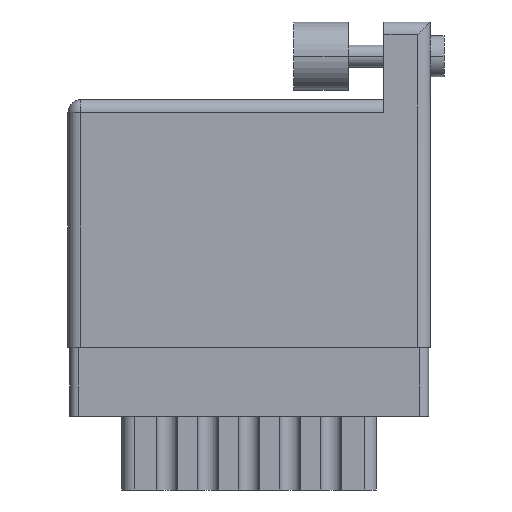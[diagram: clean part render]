
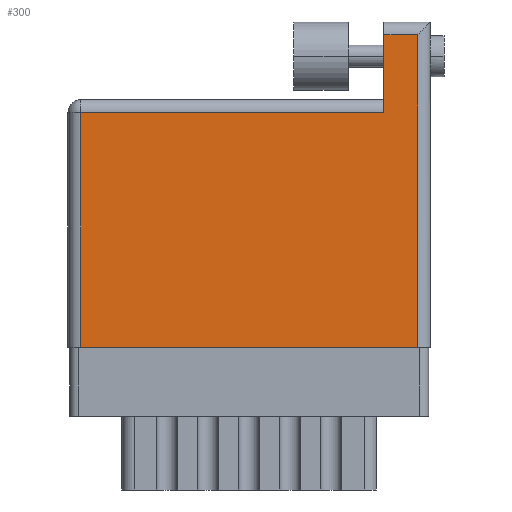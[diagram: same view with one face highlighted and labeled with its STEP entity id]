
A CAD part, front view. The second image highlights one B-rep face of the part: STEP entity #300.
In plain terms, the highlighted face is planar.
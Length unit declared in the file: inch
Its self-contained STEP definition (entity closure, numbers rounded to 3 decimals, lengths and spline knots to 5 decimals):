
#2 = EDGE_CURVE ( 'NONE', #20556, #6026, #22834, .T. ) ;
#300 = ADVANCED_FACE ( 'NONE', ( #23068 ), #21240, .F. ) ;
#415 = ORIENTED_EDGE ( 'NONE', *, *, #13060, .T. ) ;
#594 = ORIENTED_EDGE ( 'NONE', *, *, #13523, .T. ) ;
#717 = ORIENTED_EDGE ( 'NONE', *, *, #2, .T. ) ;
#747 = VERTEX_POINT ( 'NONE', #3722 ) ;
#860 = LINE ( 'NONE', #8814, #20825 ) ;
#861 = LINE ( 'NONE', #2825, #14377 ) ;
#1344 = CARTESIAN_POINT ( 'NONE',  ( 1.155, 1.143, 0. ) ) ;
#1996 = CARTESIAN_POINT ( 'NONE',  ( 1.278, 1.143, 0. ) ) ;
#2564 = DIRECTION ( 'NONE',  ( -1., 0., 0. ) ) ;
#2669 = VERTEX_POINT ( 'NONE', #22211 ) ;
#2825 = CARTESIAN_POINT ( 'NONE',  ( 0., 0.859, 0. ) ) ;
#2884 = LINE ( 'NONE', #23186, #16042 ) ;
#2885 = VERTEX_POINT ( 'NONE', #1996 ) ;
#3379 = VERTEX_POINT ( 'NONE', #1344 ) ;
#3722 = CARTESIAN_POINT ( 'NONE',  ( 0.047, 0.859, 0. ) ) ;
#4120 = VECTOR ( 'NONE', #13443, 39.37008 ) ;
#4648 = CARTESIAN_POINT ( 'NONE',  ( 0.047, 0., 0. ) ) ;
#4870 = DIRECTION ( 'NONE',  ( 1., 0., 0. ) ) ;
#5479 = CARTESIAN_POINT ( 'NONE',  ( 1.155, 1.143, 0. ) ) ;
#6026 = VERTEX_POINT ( 'NONE', #14923 ) ;
#7432 = DIRECTION ( 'NONE',  ( 0., 0., -1. ) ) ;
#8174 = EDGE_LOOP ( 'NONE', ( #717, #17718, #594, #415, #17998, #18497 ) ) ;
#8814 = CARTESIAN_POINT ( 'NONE',  ( 1.155, 1.19, 0. ) ) ;
#11611 = CARTESIAN_POINT ( 'NONE',  ( 0., 0.906, 0. ) ) ;
#13060 = EDGE_CURVE ( 'NONE', #3379, #2669, #860, .T. ) ;
#13111 = VECTOR ( 'NONE', #4870, 39.37008 ) ;
#13193 = DIRECTION ( 'NONE',  ( -1., 0., 0. ) ) ;
#13443 = DIRECTION ( 'NONE',  ( -1., 0., 0. ) ) ;
#13523 = EDGE_CURVE ( 'NONE', #2885, #3379, #23319, .T. ) ;
#14261 = EDGE_CURVE ( 'NONE', #747, #20556, #20016, .T. ) ;
#14377 = VECTOR ( 'NONE', #2564, 39.37008 ) ;
#14923 = CARTESIAN_POINT ( 'NONE',  ( 1.278, 0., 0. ) ) ;
#16042 = VECTOR ( 'NONE', #16691, 39.37008 ) ;
#16691 = DIRECTION ( 'NONE',  ( 0., 1., 0. ) ) ;
#17092 = CARTESIAN_POINT ( 'NONE',  ( 0.047, 0., 0. ) ) ;
#17718 = ORIENTED_EDGE ( 'NONE', *, *, #19200, .T. ) ;
#17998 = ORIENTED_EDGE ( 'NONE', *, *, #18498, .T. ) ;
#18497 = ORIENTED_EDGE ( 'NONE', *, *, #14261, .T. ) ;
#18498 = EDGE_CURVE ( 'NONE', #2669, #747, #861, .T. ) ;
#18980 = VECTOR ( 'NONE', #20284, 39.37008 ) ;
#19200 = EDGE_CURVE ( 'NONE', #6026, #2885, #2884, .T. ) ;
#20016 = LINE ( 'NONE', #4648, #18980 ) ;
#20284 = DIRECTION ( 'NONE',  ( 0., -1., 0. ) ) ;
#20556 = VERTEX_POINT ( 'NONE', #17092 ) ;
#20825 = VECTOR ( 'NONE', #24682, 39.37008 ) ;
#21010 = CARTESIAN_POINT ( 'NONE',  ( 0., 0., 0. ) ) ;
#21240 = PLANE ( 'NONE',  #22920 ) ;
#22211 = CARTESIAN_POINT ( 'NONE',  ( 1.155, 0.859, 0. ) ) ;
#22834 = LINE ( 'NONE', #21010, #13111 ) ;
#22920 = AXIS2_PLACEMENT_3D ( 'NONE', #11611, #7432, #13193 ) ;
#23068 = FACE_OUTER_BOUND ( 'NONE', #8174, .T. ) ;
#23186 = CARTESIAN_POINT ( 'NONE',  ( 1.278, 1.19, 0. ) ) ;
#23319 = LINE ( 'NONE', #5479, #4120 ) ;
#24682 = DIRECTION ( 'NONE',  ( 0., -1., 0. ) ) ;
